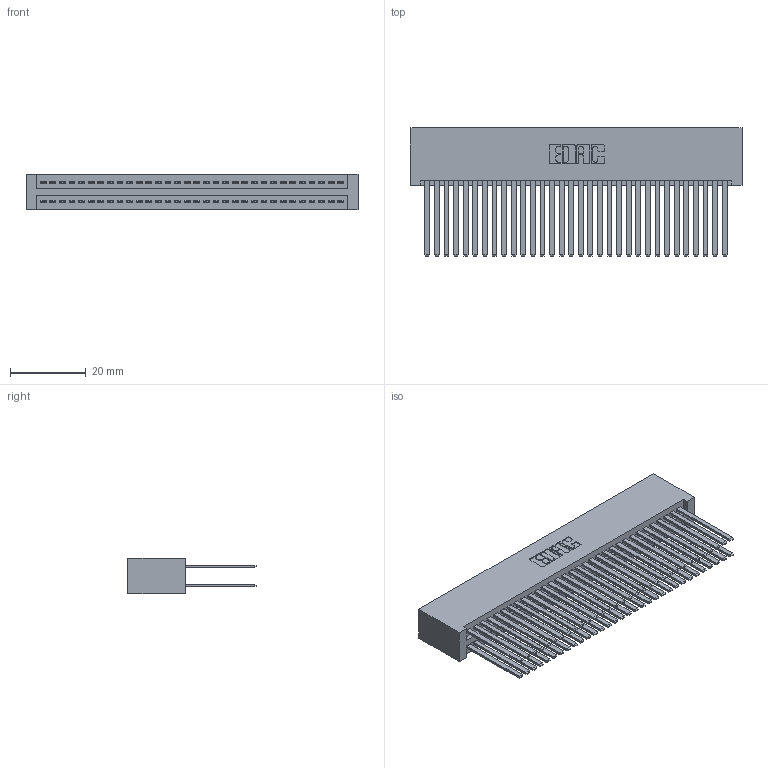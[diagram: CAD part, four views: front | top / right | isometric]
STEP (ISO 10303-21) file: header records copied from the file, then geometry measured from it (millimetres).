
FILE_DESCRIPTION (( 'STEP AP203' ), '1' );
FILE_NAME ('395-064-544-201.STEP', '2018-11-24T16:55:30', ( '' ), ( '' ), 'SwSTEP 2.0', 'SolidWorks 2016', '' );
FILE_SCHEMA (( 'CONFIG_CONTROL_DESIGN' ));
Length unit declared in the file: inch
Products named in the file (3): 345-292-001_345-293-144; 345 Part_No Mounting Lugs; 395-064-544-201
Assembly tree (65 placements, depth 2):
  395-064-544-201
    345 Part_No Mounting Lugs
    345-292-001_345-293-144  x64
Bounding box: 87.88 x 33.96 x 9.4 mm (x, y, z)
Volume: 9957.4 mm3; surface area: 17457.8 mm2
Topology: 65 solids, 65 shells, 2934 faces, 8701 edges, 5714 vertices
Faces by surface type: plane 1932, cylinder 1002
Entity records: 25993 total; most frequent: CARTESIAN_POINT 4364, ORIENTED_EDGE 4298, DIRECTION 3853, EDGE_CURVE 2149, LINE 1901, VECTOR 1901, VERTEX_POINT 1430, AXIS2_PLACEMENT_3D 976
